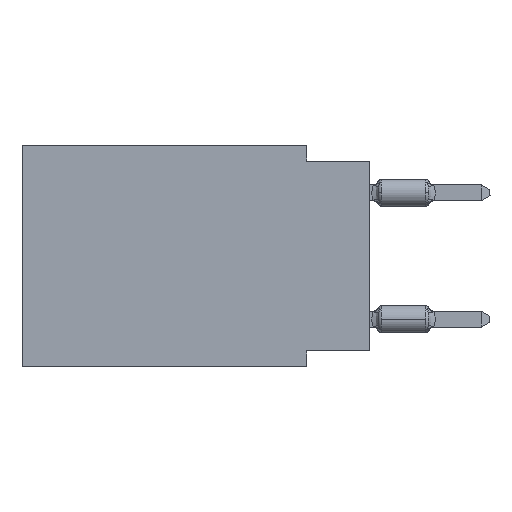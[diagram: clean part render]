
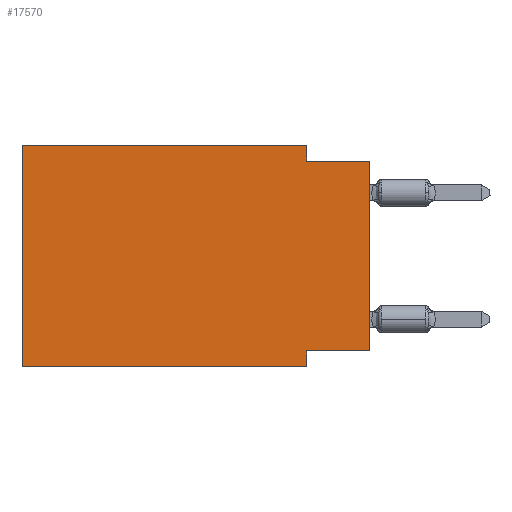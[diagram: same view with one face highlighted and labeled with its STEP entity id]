
A CAD part, left-side view. The second image highlights one B-rep face of the part: STEP entity #17570.
In plain terms, the highlighted planar face has unit normal (-1, 0, 0).
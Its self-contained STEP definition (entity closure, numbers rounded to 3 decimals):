
#1479 = VERTEX_POINT ( 'NONE', #39393 ) ;
#1858 = EDGE_CURVE ( 'NONE', #44355, #10564, #30083, .T. ) ;
#3209 = CARTESIAN_POINT ( 'NONE',  ( 0., 0., -8.255 ) ) ;
#3460 = LINE ( 'NONE', #40843, #50788 ) ;
#4474 = DIRECTION ( 'NONE',  ( 0., 0., -1. ) ) ;
#4520 = DIRECTION ( 'NONE',  ( 0., -1., 0. ) ) ;
#7070 = CARTESIAN_POINT ( 'NONE',  ( 0., 2.54, -8.89 ) ) ;
#7379 = VERTEX_POINT ( 'NONE', #44993 ) ;
#9540 = CARTESIAN_POINT ( 'NONE',  ( 0., 2.54, 0. ) ) ;
#10255 = CARTESIAN_POINT ( 'NONE',  ( 0., 2.54, 0. ) ) ;
#10440 = VERTEX_POINT ( 'NONE', #23523 ) ;
#10564 = VERTEX_POINT ( 'NONE', #11987 ) ;
#10705 = ORIENTED_EDGE ( 'NONE', *, *, #53731, .F. ) ;
#11117 = ORIENTED_EDGE ( 'NONE', *, *, #17000, .F. ) ;
#11987 = CARTESIAN_POINT ( 'NONE',  ( 0., 0., -0.635 ) ) ;
#12256 = VECTOR ( 'NONE', #34557, 1000. ) ;
#15284 = ORIENTED_EDGE ( 'NONE', *, *, #29053, .F. ) ;
#16026 = VECTOR ( 'NONE', #51939, 1000. ) ;
#16171 = EDGE_CURVE ( 'NONE', #7379, #19080, #39649, .T. ) ;
#16362 = DIRECTION ( 'NONE',  ( 0., -1., 0. ) ) ;
#17000 = EDGE_CURVE ( 'NONE', #21494, #7379, #27101, .T. ) ;
#17570 = ADVANCED_FACE ( 'NONE', ( #49725 ), #19162, .F. ) ;
#18327 = CARTESIAN_POINT ( 'NONE',  ( 0., 13.97, 0. ) ) ;
#19080 = VERTEX_POINT ( 'NONE', #10255 ) ;
#19162 = PLANE ( 'NONE',  #36837 ) ;
#21494 = VERTEX_POINT ( 'NONE', #37281 ) ;
#21596 = VECTOR ( 'NONE', #16362, 1000. ) ;
#22409 = ORIENTED_EDGE ( 'NONE', *, *, #28787, .F. ) ;
#22420 = VERTEX_POINT ( 'NONE', #7070 ) ;
#22607 = DIRECTION ( 'NONE',  ( 0., 0., 1. ) ) ;
#23523 = CARTESIAN_POINT ( 'NONE',  ( 0., 2.54, -0.635 ) ) ;
#23932 = DIRECTION ( 'NONE',  ( 1., 0., 0. ) ) ;
#25341 = LINE ( 'NONE', #51130, #21596 ) ;
#25857 = CARTESIAN_POINT ( 'NONE',  ( 0., 0., -0.635 ) ) ;
#25884 = VECTOR ( 'NONE', #4520, 1000. ) ;
#26336 = EDGE_LOOP ( 'NONE', ( #36971, #48364, #15284, #39867, #11117, #31678, #10705, #22409 ) ) ;
#26427 = CARTESIAN_POINT ( 'NONE',  ( 0., 0., 0. ) ) ;
#27101 = LINE ( 'NONE', #52351, #39375 ) ;
#27153 = EDGE_CURVE ( 'NONE', #10440, #10564, #34006, .T. ) ;
#28787 = EDGE_CURVE ( 'NONE', #44355, #1479, #31544, .T. ) ;
#29053 = EDGE_CURVE ( 'NONE', #19080, #10440, #30921, .T. ) ;
#29457 = VECTOR ( 'NONE', #4474, 1000. ) ;
#30083 = LINE ( 'NONE', #26427, #16026 ) ;
#30921 = LINE ( 'NONE', #9540, #29457 ) ;
#31535 = CARTESIAN_POINT ( 'NONE',  ( 0., 13.97, 0. ) ) ;
#31544 = LINE ( 'NONE', #53938, #54464 ) ;
#31678 = ORIENTED_EDGE ( 'NONE', *, *, #36767, .T. ) ;
#34006 = LINE ( 'NONE', #25857, #12256 ) ;
#34557 = DIRECTION ( 'NONE',  ( 0., -1., 0. ) ) ;
#36030 = DIRECTION ( 'NONE',  ( 0., 1., 0. ) ) ;
#36302 = DIRECTION ( 'NONE',  ( 0., 0., -1. ) ) ;
#36767 = EDGE_CURVE ( 'NONE', #21494, #22420, #25341, .T. ) ;
#36837 = AXIS2_PLACEMENT_3D ( 'NONE', #31535, #23932, #36302 ) ;
#36971 = ORIENTED_EDGE ( 'NONE', *, *, #1858, .T. ) ;
#37281 = CARTESIAN_POINT ( 'NONE',  ( 0., 13.97, -8.89 ) ) ;
#37757 = DIRECTION ( 'NONE',  ( 0., 0., -1. ) ) ;
#39375 = VECTOR ( 'NONE', #22607, 1000. ) ;
#39393 = CARTESIAN_POINT ( 'NONE',  ( 0., 2.54, -8.255 ) ) ;
#39649 = LINE ( 'NONE', #18327, #25884 ) ;
#39867 = ORIENTED_EDGE ( 'NONE', *, *, #16171, .F. ) ;
#40843 = CARTESIAN_POINT ( 'NONE',  ( 0., 2.54, -8.89 ) ) ;
#44355 = VERTEX_POINT ( 'NONE', #3209 ) ;
#44993 = CARTESIAN_POINT ( 'NONE',  ( 0., 13.97, 0. ) ) ;
#48364 = ORIENTED_EDGE ( 'NONE', *, *, #27153, .F. ) ;
#49725 = FACE_OUTER_BOUND ( 'NONE', #26336, .T. ) ;
#50788 = VECTOR ( 'NONE', #37757, 1000. ) ;
#51130 = CARTESIAN_POINT ( 'NONE',  ( 0., 13.97, -8.89 ) ) ;
#51939 = DIRECTION ( 'NONE',  ( 0., 0., 1. ) ) ;
#52351 = CARTESIAN_POINT ( 'NONE',  ( 0., 13.97, 0. ) ) ;
#53731 = EDGE_CURVE ( 'NONE', #1479, #22420, #3460, .T. ) ;
#53938 = CARTESIAN_POINT ( 'NONE',  ( 0., 0., -8.255 ) ) ;
#54464 = VECTOR ( 'NONE', #36030, 1000. ) ;
